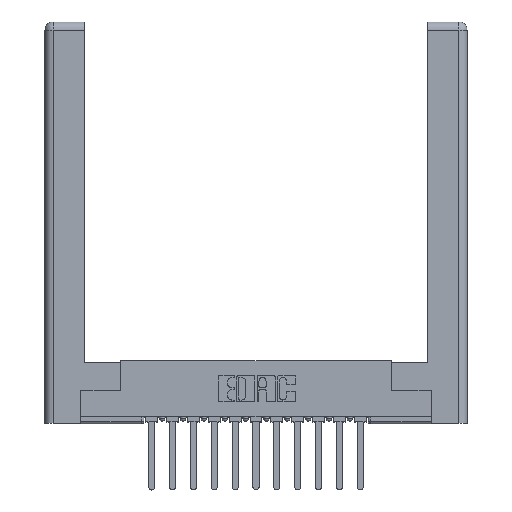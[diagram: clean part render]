
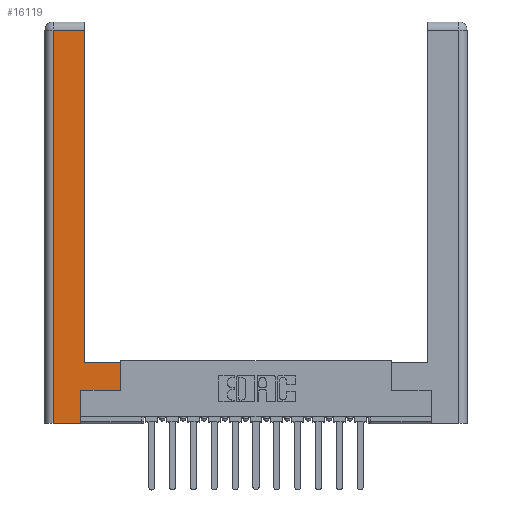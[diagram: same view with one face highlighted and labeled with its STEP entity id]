
A CAD part, top view. The second image highlights one B-rep face of the part: STEP entity #16119.
In plain terms, the highlighted planar face has unit normal (0, 0, 1).
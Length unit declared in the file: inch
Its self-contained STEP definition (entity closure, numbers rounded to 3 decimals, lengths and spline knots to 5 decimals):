
#385 = LINE ( 'NONE', #13282, #16444 ) ;
#458 = CARTESIAN_POINT ( 'NONE',  ( 0.0615, 0., 0. ) ) ;
#850 = DIRECTION ( 'NONE',  ( 0., 1., 0. ) ) ;
#1092 = DIRECTION ( 'NONE',  ( 1., 0., 0. ) ) ;
#1173 = AXIS2_PLACEMENT_3D ( 'NONE', #11351, #7368, #9933 ) ;
#1309 = VECTOR ( 'NONE', #5357, 39.37008 ) ;
#1415 = ORIENTED_EDGE ( 'NONE', *, *, #6895, .T. ) ;
#1630 = CARTESIAN_POINT ( 'NONE',  ( 0.565, 0.45, 0. ) ) ;
#1664 = EDGE_CURVE ( 'NONE', #7203, #9496, #1920, .T. ) ;
#1695 = DIRECTION ( 'NONE',  ( 0., -1., 0. ) ) ;
#1742 = EDGE_CURVE ( 'NONE', #5500, #6783, #11780, .T. ) ;
#1747 = ORIENTED_EDGE ( 'NONE', *, *, #1664, .T. ) ;
#1920 = LINE ( 'NONE', #6257, #13557 ) ;
#2050 = EDGE_CURVE ( 'NONE', #13084, #6710, #15378, .T. ) ;
#2334 = EDGE_CURVE ( 'NONE', #9496, #14986, #15957, .T. ) ;
#2417 = ORIENTED_EDGE ( 'NONE', *, *, #15242, .T. ) ;
#2758 = ORIENTED_EDGE ( 'NONE', *, *, #12520, .T. ) ;
#2777 = ORIENTED_EDGE ( 'NONE', *, *, #1742, .T. ) ;
#3296 = VECTOR ( 'NONE', #12635, 39.37008 ) ;
#4197 = VECTOR ( 'NONE', #1695, 39.37008 ) ;
#4412 = CARTESIAN_POINT ( 'NONE',  ( 0.0615, 2.94, 0. ) ) ;
#4586 = CARTESIAN_POINT ( 'NONE',  ( 0.295, 3., 0. ) ) ;
#4587 = FACE_OUTER_BOUND ( 'NONE', #13595, .T. ) ;
#5190 = CARTESIAN_POINT ( 'NONE',  ( 0.265, 0.245, 0. ) ) ;
#5210 = CARTESIAN_POINT ( 'NONE',  ( 0.295, 2.94, 0. ) ) ;
#5357 = DIRECTION ( 'NONE',  ( 0., 1., 0. ) ) ;
#5500 = VERTEX_POINT ( 'NONE', #14949 ) ;
#5514 = DIRECTION ( 'NONE',  ( -1., 0., 0. ) ) ;
#6257 = CARTESIAN_POINT ( 'NONE',  ( 0.265, 0., 0. ) ) ;
#6574 = VECTOR ( 'NONE', #5514, 39.37008 ) ;
#6710 = VERTEX_POINT ( 'NONE', #5210 ) ;
#6778 = ORIENTED_EDGE ( 'NONE', *, *, #6821, .T. ) ;
#6783 = VERTEX_POINT ( 'NONE', #1630 ) ;
#6821 = EDGE_CURVE ( 'NONE', #9591, #7203, #14622, .T. ) ;
#6895 = EDGE_CURVE ( 'NONE', #6710, #9591, #9161, .T. ) ;
#7203 = VERTEX_POINT ( 'NONE', #7260 ) ;
#7260 = CARTESIAN_POINT ( 'NONE',  ( 0.0615, 0., 0. ) ) ;
#7368 = DIRECTION ( 'NONE',  ( 0., 0., -1. ) ) ;
#9103 = LINE ( 'NONE', #16099, #3296 ) ;
#9161 = LINE ( 'NONE', #4412, #6574 ) ;
#9259 = DIRECTION ( 'NONE',  ( 0., 1., 0. ) ) ;
#9496 = VERTEX_POINT ( 'NONE', #15867 ) ;
#9591 = VERTEX_POINT ( 'NONE', #13445 ) ;
#9933 = DIRECTION ( 'NONE',  ( -1., 0., 0. ) ) ;
#10151 = VECTOR ( 'NONE', #9259, 39.37008 ) ;
#11351 = CARTESIAN_POINT ( 'NONE',  ( 0., 0., 0. ) ) ;
#11780 = LINE ( 'NONE', #14448, #10151 ) ;
#12520 = EDGE_CURVE ( 'NONE', #14986, #5500, #9103, .T. ) ;
#12605 = PLANE ( 'NONE',  #1173 ) ;
#12635 = DIRECTION ( 'NONE',  ( 1., 0., 0. ) ) ;
#12871 = ORIENTED_EDGE ( 'NONE', *, *, #2050, .T. ) ;
#13039 = CARTESIAN_POINT ( 'NONE',  ( 0.265, 0.245, 0. ) ) ;
#13084 = VERTEX_POINT ( 'NONE', #16190 ) ;
#13282 = CARTESIAN_POINT ( 'NONE',  ( 0.295, 0.45, 0. ) ) ;
#13445 = CARTESIAN_POINT ( 'NONE',  ( 0.0615, 2.94, 0. ) ) ;
#13557 = VECTOR ( 'NONE', #1092, 39.37008 ) ;
#13595 = EDGE_LOOP ( 'NONE', ( #12871, #1415, #6778, #1747, #15828, #2758, #2777, #2417 ) ) ;
#14448 = CARTESIAN_POINT ( 'NONE',  ( 0.565, 0.45, 0. ) ) ;
#14578 = DIRECTION ( 'NONE',  ( -1., 0., 0. ) ) ;
#14622 = LINE ( 'NONE', #458, #4197 ) ;
#14949 = CARTESIAN_POINT ( 'NONE',  ( 0.565, 0.245, 0. ) ) ;
#14986 = VERTEX_POINT ( 'NONE', #5190 ) ;
#15242 = EDGE_CURVE ( 'NONE', #6783, #13084, #385, .T. ) ;
#15378 = LINE ( 'NONE', #4586, #16563 ) ;
#15828 = ORIENTED_EDGE ( 'NONE', *, *, #2334, .T. ) ;
#15867 = CARTESIAN_POINT ( 'NONE',  ( 0.265, 0., 0. ) ) ;
#15957 = LINE ( 'NONE', #13039, #1309 ) ;
#16099 = CARTESIAN_POINT ( 'NONE',  ( 0.565, 0.245, 0. ) ) ;
#16119 = ADVANCED_FACE ( 'NONE', ( #4587 ), #12605, .F. ) ;
#16190 = CARTESIAN_POINT ( 'NONE',  ( 0.295, 0.45, 0. ) ) ;
#16444 = VECTOR ( 'NONE', #14578, 39.37008 ) ;
#16563 = VECTOR ( 'NONE', #850, 39.37008 ) ;
